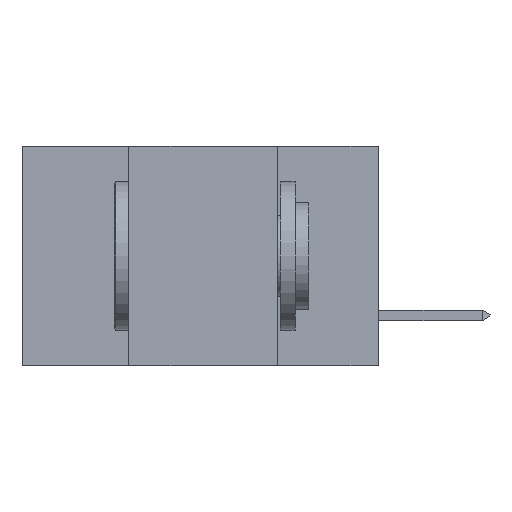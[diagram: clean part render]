
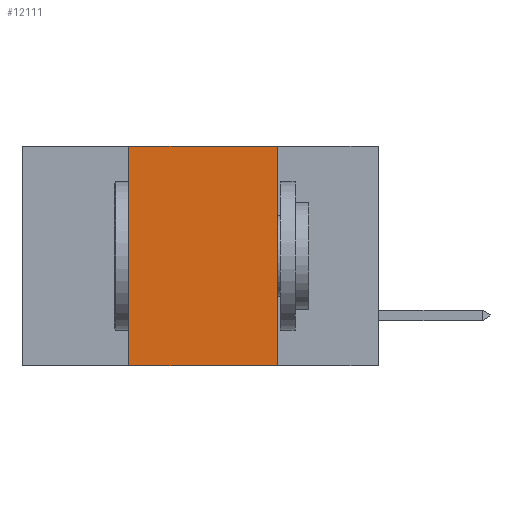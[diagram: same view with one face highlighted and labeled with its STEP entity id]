
A CAD part, left-side view. The second image highlights one B-rep face of the part: STEP entity #12111.
In plain terms, the highlighted planar face has unit normal (-1, 0, 0).
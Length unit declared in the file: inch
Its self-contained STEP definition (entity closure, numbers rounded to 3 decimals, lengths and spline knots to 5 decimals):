
#192 = PLANE ( 'NONE',  #11125 ) ;
#1059 = VERTEX_POINT ( 'NONE', #5701 ) ;
#1408 = CARTESIAN_POINT ( 'NONE',  ( 0., 0.42, 0. ) ) ;
#1564 = CARTESIAN_POINT ( 'NONE',  ( 0., 0.17, 0. ) ) ;
#1641 = VERTEX_POINT ( 'NONE', #10542 ) ;
#2861 = EDGE_LOOP ( 'NONE', ( #11168, #15887, #9536, #12775 ) ) ;
#2917 = DIRECTION ( 'NONE',  ( 1., 0., 0. ) ) ;
#3748 = DIRECTION ( 'NONE',  ( 0., 0., -1. ) ) ;
#3849 = VECTOR ( 'NONE', #3748, 39.37008 ) ;
#4161 = VERTEX_POINT ( 'NONE', #1408 ) ;
#4756 = VERTEX_POINT ( 'NONE', #1564 ) ;
#5213 = CARTESIAN_POINT ( 'NONE',  ( 0., 0.17, -0.37 ) ) ;
#5254 = LINE ( 'NONE', #6623, #10943 ) ;
#5416 = CARTESIAN_POINT ( 'NONE',  ( 0., 0.6, 0. ) ) ;
#5701 = CARTESIAN_POINT ( 'NONE',  ( 0., 0.17, -0.37 ) ) ;
#6198 = EDGE_CURVE ( 'NONE', #1641, #4161, #9568, .T. ) ;
#6623 = CARTESIAN_POINT ( 'NONE',  ( 0., 0.6, -0.37 ) ) ;
#7685 = EDGE_CURVE ( 'NONE', #4161, #4756, #14995, .T. ) ;
#8130 = CARTESIAN_POINT ( 'NONE',  ( 0., 0.6, 0. ) ) ;
#8655 = FACE_OUTER_BOUND ( 'NONE', #2861, .T. ) ;
#9377 = EDGE_CURVE ( 'NONE', #4756, #1059, #12105, .T. ) ;
#9536 = ORIENTED_EDGE ( 'NONE', *, *, #6198, .F. ) ;
#9568 = LINE ( 'NONE', #15332, #12692 ) ;
#10008 = DIRECTION ( 'NONE',  ( 0., 0., -1. ) ) ;
#10542 = CARTESIAN_POINT ( 'NONE',  ( 0., 0.42, -0.37 ) ) ;
#10781 = DIRECTION ( 'NONE',  ( 0., -1., 0. ) ) ;
#10943 = VECTOR ( 'NONE', #10781, 39.37008 ) ;
#11014 = DIRECTION ( 'NONE',  ( 0., 0., 1. ) ) ;
#11125 = AXIS2_PLACEMENT_3D ( 'NONE', #5416, #2917, #10008 ) ;
#11168 = ORIENTED_EDGE ( 'NONE', *, *, #9377, .F. ) ;
#11510 = VECTOR ( 'NONE', #13633, 39.37008 ) ;
#12105 = LINE ( 'NONE', #5213, #3849 ) ;
#12111 = ADVANCED_FACE ( 'NONE', ( #8655 ), #192, .F. ) ;
#12692 = VECTOR ( 'NONE', #11014, 39.37008 ) ;
#12775 = ORIENTED_EDGE ( 'NONE', *, *, #17799, .T. ) ;
#13633 = DIRECTION ( 'NONE',  ( 0., -1., 0. ) ) ;
#14995 = LINE ( 'NONE', #8130, #11510 ) ;
#15332 = CARTESIAN_POINT ( 'NONE',  ( 0., 0.42, -0.37 ) ) ;
#15887 = ORIENTED_EDGE ( 'NONE', *, *, #7685, .F. ) ;
#17799 = EDGE_CURVE ( 'NONE', #1641, #1059, #5254, .T. ) ;
